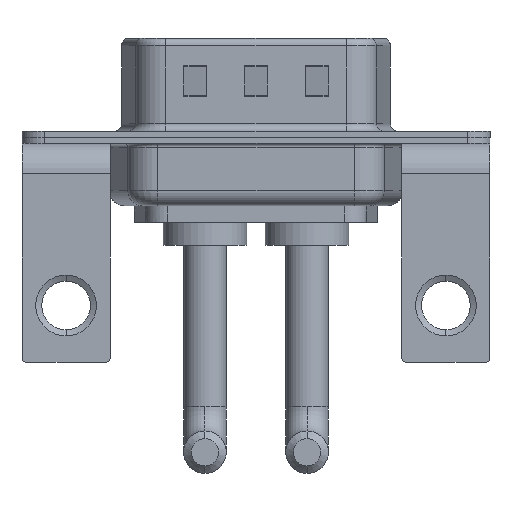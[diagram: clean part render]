
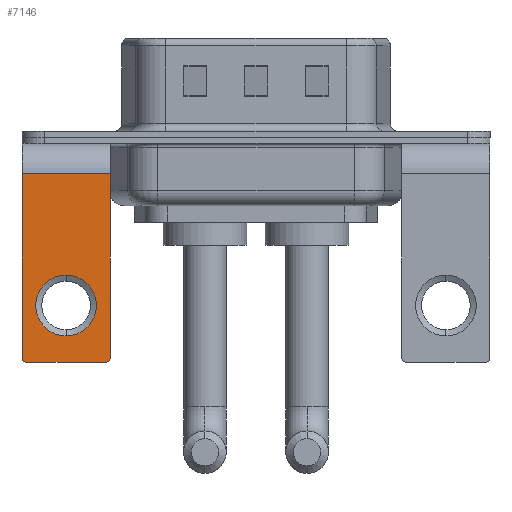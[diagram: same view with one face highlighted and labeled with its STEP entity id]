
A CAD part, front view. The second image highlights one B-rep face of the part: STEP entity #7146.
In plain terms, the highlighted planar face has unit normal (0, -1, 0).
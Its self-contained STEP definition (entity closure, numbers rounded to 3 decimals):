
#905 = LINE ( 'NONE', #9189, #5907 ) ;
#1715 = DIRECTION ( 'NONE',  ( 0., 0., 1. ) ) ;
#1755 = CARTESIAN_POINT ( 'NONE',  ( 2.9, -6.25, -2.4 ) ) ;
#1771 = VERTEX_POINT ( 'NONE', #4843 ) ;
#1852 = LINE ( 'NONE', #5299, #2025 ) ;
#2012 = AXIS2_PLACEMENT_3D ( 'NONE', #12583, #11735, #8226 ) ;
#2025 = VECTOR ( 'NONE', #3066, 1000. ) ;
#2210 = CARTESIAN_POINT ( 'NONE',  ( 0., -6.25, -9.07 ) ) ;
#2333 = LINE ( 'NONE', #9398, #5688 ) ;
#2635 = FACE_OUTER_BOUND ( 'NONE', #12175, .T. ) ;
#3066 = DIRECTION ( 'NONE',  ( 0., 0., -1. ) ) ;
#3087 = VERTEX_POINT ( 'NONE', #2210 ) ;
#3474 = ORIENTED_EDGE ( 'NONE', *, *, #11701, .F. ) ;
#3619 = EDGE_CURVE ( 'NONE', #8693, #14621, #905, .T. ) ;
#3864 = CARTESIAN_POINT ( 'NONE',  ( 2.9, -6.25, -14.8 ) ) ;
#3896 = AXIS2_PLACEMENT_3D ( 'NONE', #7384, #12257, #7688 ) ;
#4227 = CARTESIAN_POINT ( 'NONE',  ( 0., -6.25, -13.07 ) ) ;
#4448 = ORIENTED_EDGE ( 'NONE', *, *, #14094, .T. ) ;
#4705 = AXIS2_PLACEMENT_3D ( 'NONE', #12067, #7488, #7411 ) ;
#4843 = CARTESIAN_POINT ( 'NONE',  ( -2.65, -6.25, -14.8 ) ) ;
#4894 = VERTEX_POINT ( 'NONE', #14435 ) ;
#5165 = FACE_BOUND ( 'NONE', #13204, .T. ) ;
#5279 = DIRECTION ( 'NONE',  ( 0., 0., 1. ) ) ;
#5299 = CARTESIAN_POINT ( 'NONE',  ( 2.9, -6.25, -2.4 ) ) ;
#5418 = VECTOR ( 'NONE', #14373, 1000. ) ;
#5688 = VECTOR ( 'NONE', #10325, 1000. ) ;
#5907 = VECTOR ( 'NONE', #7966, 1000. ) ;
#6262 = DIRECTION ( 'NONE',  ( 0., -1., 0. ) ) ;
#6498 = EDGE_CURVE ( 'NONE', #13037, #8693, #2333, .T. ) ;
#6610 = CARTESIAN_POINT ( 'NONE',  ( 2.65, -6.25, -14.8 ) ) ;
#6834 = ORIENTED_EDGE ( 'NONE', *, *, #11276, .T. ) ;
#6841 = ORIENTED_EDGE ( 'NONE', *, *, #10252, .F. ) ;
#7146 = ADVANCED_FACE ( 'NONE', ( #5165, #2635 ), #12145, .F. ) ;
#7384 = CARTESIAN_POINT ( 'NONE',  ( 0., -6.25, -11.07 ) ) ;
#7411 = DIRECTION ( 'NONE',  ( 0., 0., 1. ) ) ;
#7488 = DIRECTION ( 'NONE',  ( 0., 1., 0. ) ) ;
#7688 = DIRECTION ( 'NONE',  ( 0., 0., 1. ) ) ;
#7966 = DIRECTION ( 'NONE',  ( 0., 0., -1. ) ) ;
#8226 = DIRECTION ( 'NONE',  ( 0., 0., 1. ) ) ;
#8578 = CARTESIAN_POINT ( 'NONE',  ( -2.65, -6.25, -14.55 ) ) ;
#8693 = VERTEX_POINT ( 'NONE', #12366 ) ;
#9166 = ORIENTED_EDGE ( 'NONE', *, *, #6498, .T. ) ;
#9189 = CARTESIAN_POINT ( 'NONE',  ( -2.9, -6.25, -2.4 ) ) ;
#9290 = EDGE_CURVE ( 'NONE', #3087, #11231, #10544, .T. ) ;
#9398 = CARTESIAN_POINT ( 'NONE',  ( 2.9, -6.25, -2.4 ) ) ;
#9626 = CARTESIAN_POINT ( 'NONE',  ( 2.65, -6.25, -14.55 ) ) ;
#9938 = CIRCLE ( 'NONE', #11879, 0.25 ) ;
#10252 = EDGE_CURVE ( 'NONE', #12515, #1771, #10873, .T. ) ;
#10325 = DIRECTION ( 'NONE',  ( -1., 0., 0. ) ) ;
#10544 = CIRCLE ( 'NONE', #3896, 2. ) ;
#10873 = LINE ( 'NONE', #3864, #5418 ) ;
#11108 = DIRECTION ( 'NONE',  ( 0., -1., 0. ) ) ;
#11231 = VERTEX_POINT ( 'NONE', #4227 ) ;
#11276 = EDGE_CURVE ( 'NONE', #11231, #3087, #13512, .T. ) ;
#11491 = CARTESIAN_POINT ( 'NONE',  ( -2.9, -6.25, -14.55 ) ) ;
#11701 = EDGE_CURVE ( 'NONE', #13037, #4894, #1852, .T. ) ;
#11735 = DIRECTION ( 'NONE',  ( 0., 1., 0. ) ) ;
#11879 = AXIS2_PLACEMENT_3D ( 'NONE', #9626, #6262, #1715 ) ;
#11898 = ORIENTED_EDGE ( 'NONE', *, *, #3619, .T. ) ;
#12067 = CARTESIAN_POINT ( 'NONE',  ( 2.9, -6.25, -2.4 ) ) ;
#12141 = ORIENTED_EDGE ( 'NONE', *, *, #9290, .T. ) ;
#12145 = PLANE ( 'NONE',  #4705 ) ;
#12175 = EDGE_LOOP ( 'NONE', ( #11898, #13268, #6841, #4448, #3474, #9166 ) ) ;
#12257 = DIRECTION ( 'NONE',  ( 0., 1., 0. ) ) ;
#12366 = CARTESIAN_POINT ( 'NONE',  ( -2.9, -6.25, -2.4 ) ) ;
#12515 = VERTEX_POINT ( 'NONE', #6610 ) ;
#12573 = CIRCLE ( 'NONE', #14523, 0.25 ) ;
#12583 = CARTESIAN_POINT ( 'NONE',  ( 0., -6.25, -11.07 ) ) ;
#13037 = VERTEX_POINT ( 'NONE', #1755 ) ;
#13105 = EDGE_CURVE ( 'NONE', #14621, #1771, #12573, .T. ) ;
#13204 = EDGE_LOOP ( 'NONE', ( #6834, #12141 ) ) ;
#13268 = ORIENTED_EDGE ( 'NONE', *, *, #13105, .T. ) ;
#13512 = CIRCLE ( 'NONE', #2012, 2. ) ;
#14094 = EDGE_CURVE ( 'NONE', #12515, #4894, #9938, .T. ) ;
#14373 = DIRECTION ( 'NONE',  ( -1., 0., 0. ) ) ;
#14435 = CARTESIAN_POINT ( 'NONE',  ( 2.9, -6.25, -14.55 ) ) ;
#14523 = AXIS2_PLACEMENT_3D ( 'NONE', #8578, #11108, #5279 ) ;
#14621 = VERTEX_POINT ( 'NONE', #11491 ) ;
